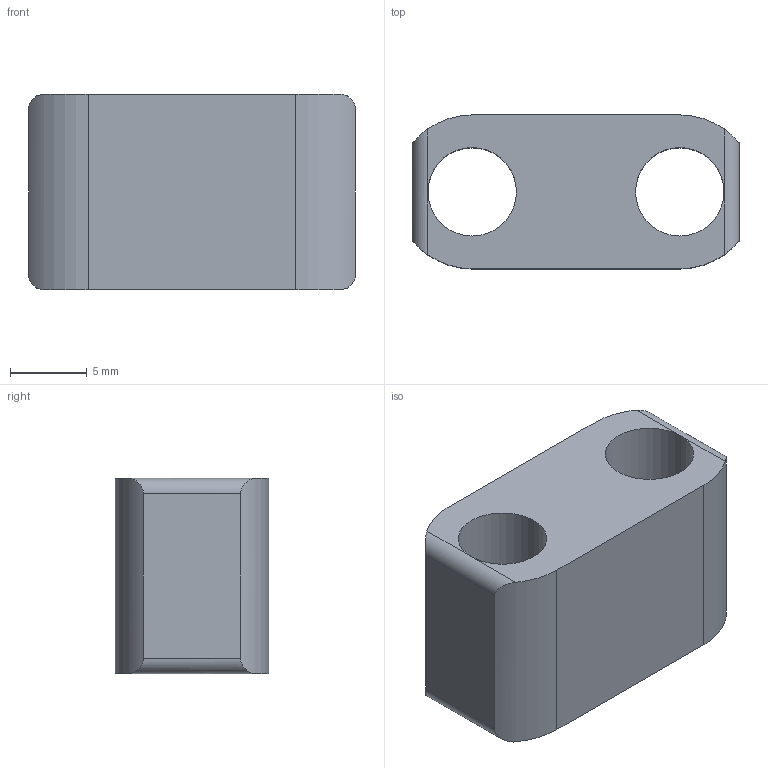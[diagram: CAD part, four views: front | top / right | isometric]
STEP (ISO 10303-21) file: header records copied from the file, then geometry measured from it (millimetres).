
FILE_DESCRIPTION (( 'STEP AP203' ), '1' );
FILE_NAME ('BufferToFCGMid.STEP', '2019-09-03T07:06:28', ( '' ), ( '' ), 'SwSTEP 2.0', 'SolidWorks 2018', '' );
FILE_SCHEMA (( 'CONFIG_CONTROL_DESIGN' ));
Length unit declared in the file: millimetre
Products named in the file (1): BufferToFCGMid
Bounding box: 21.25 x 10 x 12.7 mm (x, y, z)
Volume: 1923.2 mm3; surface area: 1478.5 mm2
Topology: 1 solids, 1 shells, 18 faces, 52 edges, 32 vertices
Faces by surface type: cylinder 12, plane 6
Entity records: 729 total; most frequent: CARTESIAN_POINT 175, ORIENTED_EDGE 104, DIRECTION 98, EDGE_CURVE 52, AXIS2_PLACEMENT_3D 35, VERTEX_POINT 32, LINE 28, VECTOR 28
